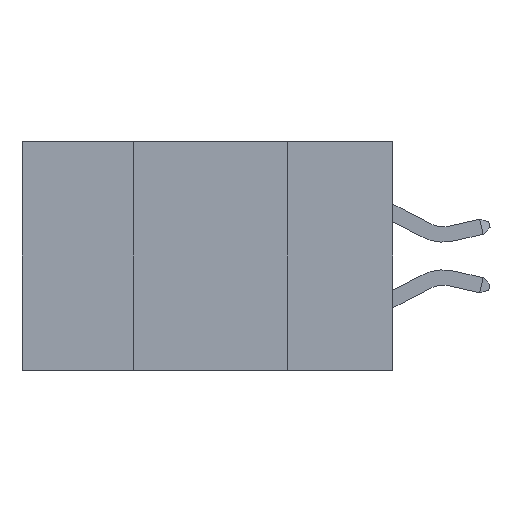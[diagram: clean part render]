
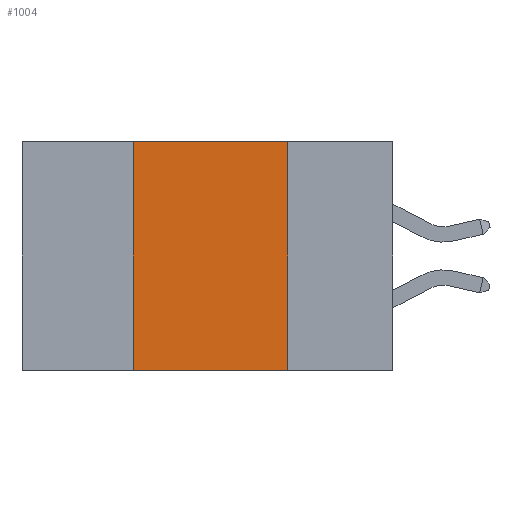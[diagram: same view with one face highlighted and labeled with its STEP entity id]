
A CAD part, left-side view. The second image highlights one B-rep face of the part: STEP entity #1004.
In plain terms, the highlighted planar face has unit normal (-1, 0, 0).
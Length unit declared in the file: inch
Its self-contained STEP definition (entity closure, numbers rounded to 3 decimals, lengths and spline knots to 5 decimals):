
#52 = VECTOR ( 'NONE', #1760, 39.37008 ) ;
#246 = VECTOR ( 'NONE', #1204, 39.37008 ) ;
#413 = ORIENTED_EDGE ( 'NONE', *, *, #8163, .T. ) ;
#1004 = ADVANCED_FACE ( 'NONE', ( #1266 ), #3787, .F. ) ;
#1029 = CARTESIAN_POINT ( 'NONE',  ( 0., 0.6, 0. ) ) ;
#1204 = DIRECTION ( 'NONE',  ( 0., -1., 0. ) ) ;
#1266 = FACE_OUTER_BOUND ( 'NONE', #1925, .T. ) ;
#1520 = EDGE_CURVE ( 'NONE', #5875, #8578, #6192, .T. ) ;
#1760 = DIRECTION ( 'NONE',  ( 0., 0., 1. ) ) ;
#1925 = EDGE_LOOP ( 'NONE', ( #9157, #4247, #8162, #413 ) ) ;
#2127 = DIRECTION ( 'NONE',  ( 0., -1., 0. ) ) ;
#3594 = CARTESIAN_POINT ( 'NONE',  ( 0., 0.17, 0. ) ) ;
#3612 = VECTOR ( 'NONE', #2127, 39.37008 ) ;
#3642 = CARTESIAN_POINT ( 'NONE',  ( 0., 0.17, 0. ) ) ;
#3737 = VERTEX_POINT ( 'NONE', #5261 ) ;
#3787 = PLANE ( 'NONE',  #7100 ) ;
#4247 = ORIENTED_EDGE ( 'NONE', *, *, #4750, .F. ) ;
#4469 = VECTOR ( 'NONE', #9017, 39.37008 ) ;
#4750 = EDGE_CURVE ( 'NONE', #7483, #5875, #7992, .T. ) ;
#5261 = CARTESIAN_POINT ( 'NONE',  ( 0., 0.42, -0.37 ) ) ;
#5368 = CARTESIAN_POINT ( 'NONE',  ( 0., 0.6, 0. ) ) ;
#5428 = CARTESIAN_POINT ( 'NONE',  ( 0., 0.42, 0. ) ) ;
#5875 = VERTEX_POINT ( 'NONE', #3594 ) ;
#5905 = DIRECTION ( 'NONE',  ( 0., 0., -1. ) ) ;
#6003 = DIRECTION ( 'NONE',  ( 1., 0., 0. ) ) ;
#6192 = LINE ( 'NONE', #3642, #4469 ) ;
#7100 = AXIS2_PLACEMENT_3D ( 'NONE', #5368, #6003, #5905 ) ;
#7124 = CARTESIAN_POINT ( 'NONE',  ( 0., 0.17, -0.37 ) ) ;
#7483 = VERTEX_POINT ( 'NONE', #8387 ) ;
#7992 = LINE ( 'NONE', #1029, #246 ) ;
#8162 = ORIENTED_EDGE ( 'NONE', *, *, #9010, .F. ) ;
#8163 = EDGE_CURVE ( 'NONE', #3737, #8578, #9230, .T. ) ;
#8387 = CARTESIAN_POINT ( 'NONE',  ( 0., 0.42, 0. ) ) ;
#8578 = VERTEX_POINT ( 'NONE', #7124 ) ;
#9010 = EDGE_CURVE ( 'NONE', #3737, #7483, #9115, .T. ) ;
#9017 = DIRECTION ( 'NONE',  ( 0., 0., -1. ) ) ;
#9115 = LINE ( 'NONE', #5428, #52 ) ;
#9157 = ORIENTED_EDGE ( 'NONE', *, *, #1520, .F. ) ;
#9220 = CARTESIAN_POINT ( 'NONE',  ( 0., 0.6, -0.37 ) ) ;
#9230 = LINE ( 'NONE', #9220, #3612 ) ;
